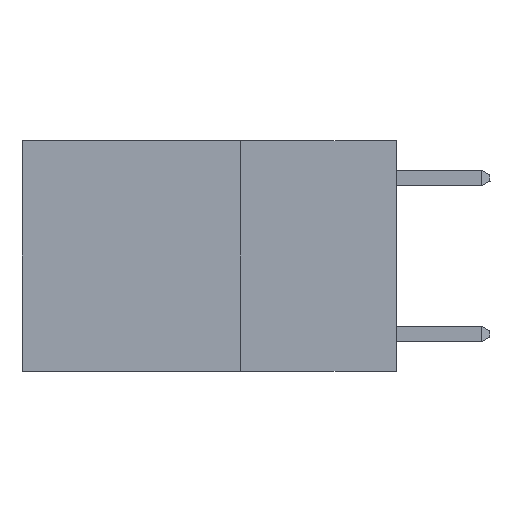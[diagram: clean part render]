
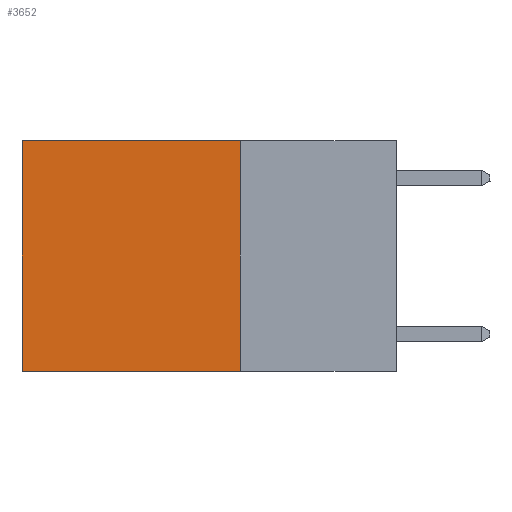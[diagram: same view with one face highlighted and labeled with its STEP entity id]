
A CAD part, left-side view. The second image highlights one B-rep face of the part: STEP entity #3652.
In plain terms, the highlighted planar face has unit normal (-1, 0, 0).
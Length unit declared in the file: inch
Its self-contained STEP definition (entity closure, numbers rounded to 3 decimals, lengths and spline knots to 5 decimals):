
#4 = DIRECTION ( 'NONE',  ( 0., 0., -1. ) ) ;
#443 = VERTEX_POINT ( 'NONE', #13753 ) ;
#462 = EDGE_CURVE ( 'NONE', #443, #9067, #4916, .T. ) ;
#492 = VECTOR ( 'NONE', #5661, 39.37008 ) ;
#914 = AXIS2_PLACEMENT_3D ( 'NONE', #8175, #12779, #5840 ) ;
#1475 = VECTOR ( 'NONE', #11481, 39.37008 ) ;
#1805 = PLANE ( 'NONE',  #914 ) ;
#3097 = CARTESIAN_POINT ( 'NONE',  ( 0.2625, 0.6, -0.37 ) ) ;
#3652 = ADVANCED_FACE ( 'NONE', ( #4173 ), #1805, .F. ) ;
#3969 = LINE ( 'NONE', #4320, #492 ) ;
#4173 = FACE_OUTER_BOUND ( 'NONE', #9460, .T. ) ;
#4320 = CARTESIAN_POINT ( 'NONE',  ( 0.2625, 0.25, 0. ) ) ;
#4916 = LINE ( 'NONE', #10438, #13507 ) ;
#5661 = DIRECTION ( 'NONE',  ( 0., 1., 0. ) ) ;
#5840 = DIRECTION ( 'NONE',  ( 0., 0., -1. ) ) ;
#5952 = VERTEX_POINT ( 'NONE', #9180 ) ;
#6194 = DIRECTION ( 'NONE',  ( 0., 0., -1. ) ) ;
#7363 = ORIENTED_EDGE ( 'NONE', *, *, #462, .T. ) ;
#7509 = ORIENTED_EDGE ( 'NONE', *, *, #8063, .F. ) ;
#7525 = ORIENTED_EDGE ( 'NONE', *, *, #14372, .F. ) ;
#7662 = ORIENTED_EDGE ( 'NONE', *, *, #8979, .T. ) ;
#8063 = EDGE_CURVE ( 'NONE', #5952, #9067, #11701, .T. ) ;
#8175 = CARTESIAN_POINT ( 'NONE',  ( 0.2625, 0.25, 0. ) ) ;
#8192 = CARTESIAN_POINT ( 'NONE',  ( 0.2625, 0.25, 0. ) ) ;
#8979 = EDGE_CURVE ( 'NONE', #10049, #443, #3969, .T. ) ;
#9067 = VERTEX_POINT ( 'NONE', #3097 ) ;
#9180 = CARTESIAN_POINT ( 'NONE',  ( 0.2625, 0.25, -0.37 ) ) ;
#9460 = EDGE_LOOP ( 'NONE', ( #7363, #7509, #7525, #7662 ) ) ;
#10049 = VERTEX_POINT ( 'NONE', #8192 ) ;
#10349 = CARTESIAN_POINT ( 'NONE',  ( 0.2625, 0.25, -0.37 ) ) ;
#10438 = CARTESIAN_POINT ( 'NONE',  ( 0.2625, 0.6, 0. ) ) ;
#11481 = DIRECTION ( 'NONE',  ( 0., 1., 0. ) ) ;
#11701 = LINE ( 'NONE', #10349, #1475 ) ;
#12779 = DIRECTION ( 'NONE',  ( 1., 0., 0. ) ) ;
#13507 = VECTOR ( 'NONE', #6194, 39.37008 ) ;
#13753 = CARTESIAN_POINT ( 'NONE',  ( 0.2625, 0.6, 0. ) ) ;
#14344 = VECTOR ( 'NONE', #4, 39.37008 ) ;
#14372 = EDGE_CURVE ( 'NONE', #10049, #5952, #14686, .T. ) ;
#14475 = CARTESIAN_POINT ( 'NONE',  ( 0.2625, 0.25, 0. ) ) ;
#14686 = LINE ( 'NONE', #14475, #14344 ) ;
